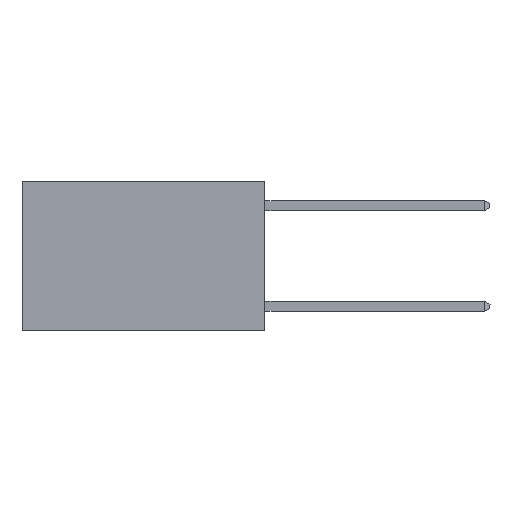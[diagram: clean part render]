
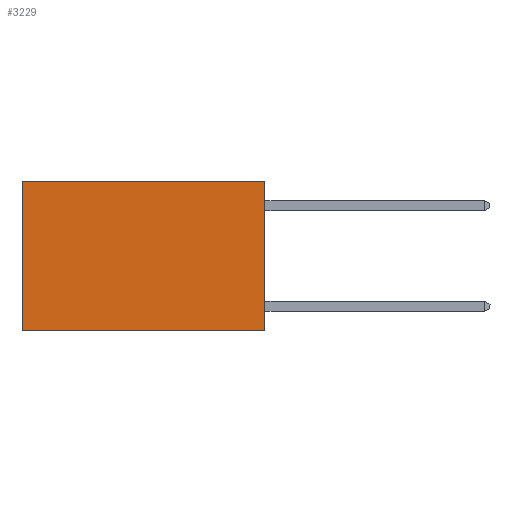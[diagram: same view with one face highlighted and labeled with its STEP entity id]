
A CAD part, left-side view. The second image highlights one B-rep face of the part: STEP entity #3229.
In plain terms, the highlighted planar face has unit normal (-1, 0, 0).
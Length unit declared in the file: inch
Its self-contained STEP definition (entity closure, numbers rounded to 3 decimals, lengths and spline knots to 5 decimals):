
#333 = DIRECTION ( 'NONE',  ( 0., 1., 0. ) ) ;
#465 = LINE ( 'NONE', #2551, #2539 ) ;
#865 = CARTESIAN_POINT ( 'NONE',  ( 0.2625, 0.6, -0.37 ) ) ;
#972 = PLANE ( 'NONE',  #9485 ) ;
#1217 = VERTEX_POINT ( 'NONE', #8671 ) ;
#1247 = VERTEX_POINT ( 'NONE', #865 ) ;
#1464 = DIRECTION ( 'NONE',  ( 0., 0., -1. ) ) ;
#1609 = VERTEX_POINT ( 'NONE', #14171 ) ;
#2090 = DIRECTION ( 'NONE',  ( 0., 0., -1. ) ) ;
#2471 = CARTESIAN_POINT ( 'NONE',  ( 0.2625, 0., -0.37 ) ) ;
#2539 = VECTOR ( 'NONE', #1464, 39.37008 ) ;
#2551 = CARTESIAN_POINT ( 'NONE',  ( 0.2625, 0.6, 0. ) ) ;
#3229 = ADVANCED_FACE ( 'NONE', ( #6212 ), #972, .F. ) ;
#3306 = EDGE_CURVE ( 'NONE', #3569, #1217, #8398, .T. ) ;
#3569 = VERTEX_POINT ( 'NONE', #3766 ) ;
#3766 = CARTESIAN_POINT ( 'NONE',  ( 0.2625, 0., 0. ) ) ;
#4018 = VECTOR ( 'NONE', #8871, 39.37008 ) ;
#4200 = EDGE_CURVE ( 'NONE', #1609, #1247, #6531, .T. ) ;
#4616 = ORIENTED_EDGE ( 'NONE', *, *, #12691, .T. ) ;
#5403 = CARTESIAN_POINT ( 'NONE',  ( 0.2625, 0., 0. ) ) ;
#5713 = CARTESIAN_POINT ( 'NONE',  ( 0.2625, 0., 0. ) ) ;
#6212 = FACE_OUTER_BOUND ( 'NONE', #12478, .T. ) ;
#6465 = DIRECTION ( 'NONE',  ( 0., 0., -1. ) ) ;
#6531 = LINE ( 'NONE', #2471, #13583 ) ;
#7536 = DIRECTION ( 'NONE',  ( 1., 0., 0. ) ) ;
#8036 = EDGE_CURVE ( 'NONE', #3569, #1609, #9038, .T. ) ;
#8398 = LINE ( 'NONE', #5713, #4018 ) ;
#8671 = CARTESIAN_POINT ( 'NONE',  ( 0.2625, 0.6, 0. ) ) ;
#8871 = DIRECTION ( 'NONE',  ( 0., 1., 0. ) ) ;
#8881 = ORIENTED_EDGE ( 'NONE', *, *, #4200, .F. ) ;
#9038 = LINE ( 'NONE', #9677, #11667 ) ;
#9485 = AXIS2_PLACEMENT_3D ( 'NONE', #5403, #7536, #6465 ) ;
#9677 = CARTESIAN_POINT ( 'NONE',  ( 0.2625, 0., 0. ) ) ;
#11667 = VECTOR ( 'NONE', #2090, 39.37008 ) ;
#12288 = ORIENTED_EDGE ( 'NONE', *, *, #8036, .F. ) ;
#12478 = EDGE_LOOP ( 'NONE', ( #4616, #8881, #12288, #13091 ) ) ;
#12691 = EDGE_CURVE ( 'NONE', #1217, #1247, #465, .T. ) ;
#13091 = ORIENTED_EDGE ( 'NONE', *, *, #3306, .T. ) ;
#13583 = VECTOR ( 'NONE', #333, 39.37008 ) ;
#14171 = CARTESIAN_POINT ( 'NONE',  ( 0.2625, 0., -0.37 ) ) ;
